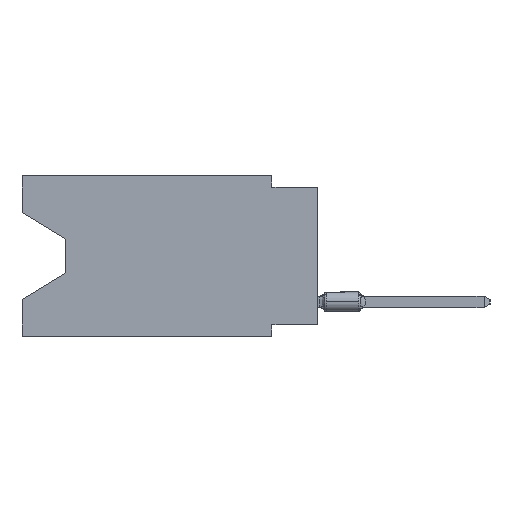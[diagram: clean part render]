
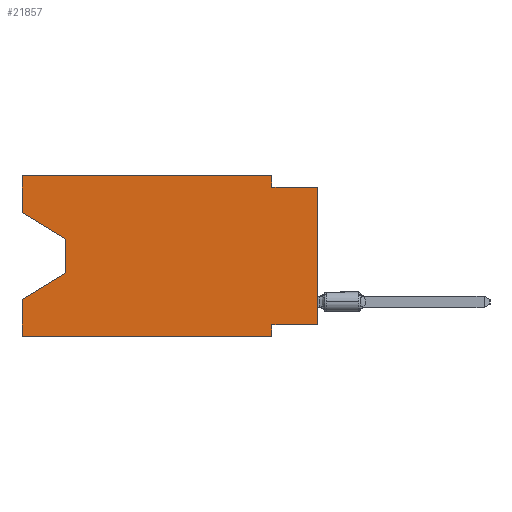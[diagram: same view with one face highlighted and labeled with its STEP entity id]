
A CAD part, left-side view. The second image highlights one B-rep face of the part: STEP entity #21857.
In plain terms, the highlighted planar face has unit normal (-1, 0, 0).
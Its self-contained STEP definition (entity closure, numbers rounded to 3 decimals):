
#298 = CARTESIAN_POINT ( 'NONE',  ( 0., 0., -0.635 ) ) ;
#645 = EDGE_CURVE ( 'NONE', #34786, #30942, #52521, .T. ) ;
#1147 = CARTESIAN_POINT ( 'NONE',  ( 0., 16.383, 0. ) ) ;
#1533 = LINE ( 'NONE', #6831, #12216 ) ;
#1732 = CARTESIAN_POINT ( 'NONE',  ( 0., 2.54, -8.89 ) ) ;
#1908 = EDGE_CURVE ( 'NONE', #34786, #3869, #27723, .T. ) ;
#3869 = VERTEX_POINT ( 'NONE', #43213 ) ;
#4918 = EDGE_CURVE ( 'NONE', #45357, #24279, #34225, .T. ) ;
#5727 = DIRECTION ( 'NONE',  ( 0., -0.855, -0.519 ) ) ;
#5796 = LINE ( 'NONE', #13788, #57318 ) ;
#6659 = ORIENTED_EDGE ( 'NONE', *, *, #28388, .F. ) ;
#6782 = CARTESIAN_POINT ( 'NONE',  ( 0., 2.54, -8.255 ) ) ;
#6826 = CARTESIAN_POINT ( 'NONE',  ( 0., 13.97, -3.505 ) ) ;
#6831 = CARTESIAN_POINT ( 'NONE',  ( 0., 13.97, -5.385 ) ) ;
#8308 = PLANE ( 'NONE',  #11027 ) ;
#8554 = DIRECTION ( 'NONE',  ( 0., -1., 0. ) ) ;
#10822 = VERTEX_POINT ( 'NONE', #41040 ) ;
#10858 = CARTESIAN_POINT ( 'NONE',  ( 0., 13.97, -3.505 ) ) ;
#11027 = AXIS2_PLACEMENT_3D ( 'NONE', #48424, #26615, #17451 ) ;
#12127 = LINE ( 'NONE', #52244, #31095 ) ;
#12216 = VECTOR ( 'NONE', #24833, 1000. ) ;
#13788 = CARTESIAN_POINT ( 'NONE',  ( 0., 2.54, 0. ) ) ;
#14793 = LINE ( 'NONE', #45494, #48516 ) ;
#15188 = VECTOR ( 'NONE', #46940, 1000. ) ;
#16240 = ORIENTED_EDGE ( 'NONE', *, *, #41604, .T. ) ;
#16512 = CARTESIAN_POINT ( 'NONE',  ( 0., 0., -0.635 ) ) ;
#16921 = VERTEX_POINT ( 'NONE', #20716 ) ;
#17451 = DIRECTION ( 'NONE',  ( 0., 0., -1. ) ) ;
#17643 = DIRECTION ( 'NONE',  ( 0., 0., -1. ) ) ;
#19138 = DIRECTION ( 'NONE',  ( 0., 0., 1. ) ) ;
#20215 = VECTOR ( 'NONE', #28586, 1000. ) ;
#20716 = CARTESIAN_POINT ( 'NONE',  ( 0., 2.54, 0. ) ) ;
#21608 = VERTEX_POINT ( 'NONE', #57705 ) ;
#21857 = ADVANCED_FACE ( 'NONE', ( #43711 ), #8308, .F. ) ;
#23797 = DIRECTION ( 'NONE',  ( 0., 0., -1. ) ) ;
#24026 = ORIENTED_EDGE ( 'NONE', *, *, #53388, .F. ) ;
#24279 = VERTEX_POINT ( 'NONE', #298 ) ;
#24833 = DIRECTION ( 'NONE',  ( 0., 0.855, -0.519 ) ) ;
#24857 = ORIENTED_EDGE ( 'NONE', *, *, #1908, .F. ) ;
#26521 = EDGE_CURVE ( 'NONE', #10822, #56406, #12127, .T. ) ;
#26532 = VERTEX_POINT ( 'NONE', #6826 ) ;
#26615 = DIRECTION ( 'NONE',  ( 1., 0., 0. ) ) ;
#27723 = LINE ( 'NONE', #1147, #36587 ) ;
#28388 = EDGE_CURVE ( 'NONE', #16921, #45357, #5796, .T. ) ;
#28586 = DIRECTION ( 'NONE',  ( 0., 0., -1. ) ) ;
#29076 = ORIENTED_EDGE ( 'NONE', *, *, #26521, .F. ) ;
#29337 = ORIENTED_EDGE ( 'NONE', *, *, #4918, .F. ) ;
#29369 = EDGE_CURVE ( 'NONE', #32956, #3869, #1533, .T. ) ;
#29553 = LINE ( 'NONE', #37805, #15188 ) ;
#30942 = VERTEX_POINT ( 'NONE', #1732 ) ;
#31095 = VECTOR ( 'NONE', #34263, 1000. ) ;
#32226 = DIRECTION ( 'NONE',  ( 0., 0., 1. ) ) ;
#32724 = EDGE_LOOP ( 'NONE', ( #44781, #44984, #53830, #24857, #51941, #56002, #29076, #16240, #29337, #6659, #24026, #56971 ) ) ;
#32956 = VERTEX_POINT ( 'NONE', #55827 ) ;
#34225 = LINE ( 'NONE', #16512, #56483 ) ;
#34263 = DIRECTION ( 'NONE',  ( 0., 1., 0. ) ) ;
#34786 = VERTEX_POINT ( 'NONE', #56065 ) ;
#35113 = EDGE_CURVE ( 'NONE', #26532, #32956, #37999, .T. ) ;
#36587 = VECTOR ( 'NONE', #19138, 1000. ) ;
#37152 = CARTESIAN_POINT ( 'NONE',  ( 0., 16.383, -2.038 ) ) ;
#37805 = CARTESIAN_POINT ( 'NONE',  ( 0., 16.383, 0. ) ) ;
#37999 = LINE ( 'NONE', #10858, #20215 ) ;
#40059 = LINE ( 'NONE', #58050, #47246 ) ;
#40449 = DIRECTION ( 'NONE',  ( 0., -1., 0. ) ) ;
#41040 = CARTESIAN_POINT ( 'NONE',  ( 0., 0., -8.255 ) ) ;
#41604 = EDGE_CURVE ( 'NONE', #10822, #24279, #14793, .T. ) ;
#41986 = LINE ( 'NONE', #49184, #57543 ) ;
#43213 = CARTESIAN_POINT ( 'NONE',  ( 0., 16.383, -6.852 ) ) ;
#43395 = CARTESIAN_POINT ( 'NONE',  ( 0., 16.383, -8.89 ) ) ;
#43711 = FACE_OUTER_BOUND ( 'NONE', #32724, .T. ) ;
#44781 = ORIENTED_EDGE ( 'NONE', *, *, #49645, .T. ) ;
#44984 = ORIENTED_EDGE ( 'NONE', *, *, #35113, .T. ) ;
#45357 = VERTEX_POINT ( 'NONE', #50996 ) ;
#45494 = CARTESIAN_POINT ( 'NONE',  ( 0., 0., 0. ) ) ;
#46940 = DIRECTION ( 'NONE',  ( 0., 0., 1. ) ) ;
#47226 = DIRECTION ( 'NONE',  ( 0., -1., 0. ) ) ;
#47246 = VECTOR ( 'NONE', #17643, 1000. ) ;
#48424 = CARTESIAN_POINT ( 'NONE',  ( 0., 16.383, 0. ) ) ;
#48516 = VECTOR ( 'NONE', #32226, 1000. ) ;
#49014 = CARTESIAN_POINT ( 'NONE',  ( 0., 16.383, 0. ) ) ;
#49184 = CARTESIAN_POINT ( 'NONE',  ( 0., 16.383, -2.038 ) ) ;
#49645 = EDGE_CURVE ( 'NONE', #50426, #26532, #41986, .T. ) ;
#50205 = EDGE_CURVE ( 'NONE', #50426, #21608, #29553, .T. ) ;
#50426 = VERTEX_POINT ( 'NONE', #37152 ) ;
#50713 = EDGE_CURVE ( 'NONE', #56406, #30942, #40059, .T. ) ;
#50996 = CARTESIAN_POINT ( 'NONE',  ( 0., 2.54, -0.635 ) ) ;
#51941 = ORIENTED_EDGE ( 'NONE', *, *, #645, .T. ) ;
#52244 = CARTESIAN_POINT ( 'NONE',  ( 0., 0., -8.255 ) ) ;
#52521 = LINE ( 'NONE', #43395, #54643 ) ;
#53388 = EDGE_CURVE ( 'NONE', #21608, #16921, #54005, .T. ) ;
#53830 = ORIENTED_EDGE ( 'NONE', *, *, #29369, .T. ) ;
#54005 = LINE ( 'NONE', #49014, #54913 ) ;
#54643 = VECTOR ( 'NONE', #47226, 1000. ) ;
#54913 = VECTOR ( 'NONE', #40449, 1000. ) ;
#55827 = CARTESIAN_POINT ( 'NONE',  ( 0., 13.97, -5.385 ) ) ;
#56002 = ORIENTED_EDGE ( 'NONE', *, *, #50713, .F. ) ;
#56065 = CARTESIAN_POINT ( 'NONE',  ( 0., 16.383, -8.89 ) ) ;
#56406 = VERTEX_POINT ( 'NONE', #6782 ) ;
#56483 = VECTOR ( 'NONE', #8554, 1000. ) ;
#56971 = ORIENTED_EDGE ( 'NONE', *, *, #50205, .F. ) ;
#57318 = VECTOR ( 'NONE', #23797, 1000. ) ;
#57543 = VECTOR ( 'NONE', #5727, 1000. ) ;
#57705 = CARTESIAN_POINT ( 'NONE',  ( 0., 16.383, 0. ) ) ;
#58050 = CARTESIAN_POINT ( 'NONE',  ( 0., 2.54, -8.89 ) ) ;
